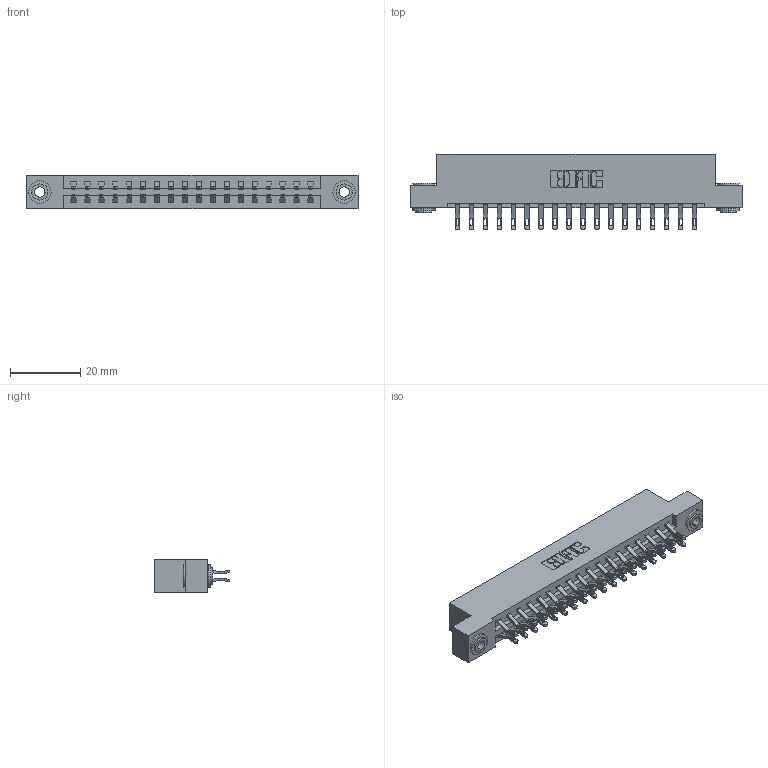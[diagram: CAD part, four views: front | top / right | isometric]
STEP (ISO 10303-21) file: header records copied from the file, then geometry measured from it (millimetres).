
FILE_DESCRIPTION (( 'STEP AP203' ), '1' );
FILE_NAME ('337-036-555-203.STEP', '2019-10-08T21:03:38', ( '' ), ( '' ), 'SwSTEP 2.0', 'SolidWorks 2016', '' );
FILE_SCHEMA (( 'CONFIG_CONTROL_DESIGN' ));
Length unit declared in the file: inch
Products named in the file (4): 345-292-001_555 Tail; 337 Part_Flush Mounting Lugs - 0.156 Dia-TH; 345-250-002_345-250-002-102; 337-036-555-203
Assembly tree (39 placements, depth 2):
  337-036-555-203
    337 Part_Flush Mounting Lugs - 0.156 Dia-TH
    345-292-001_555 Tail  x36
    345-250-002_345-250-002-102  x2
Bounding box: 94.34 x 21.47 x 9.4 mm (x, y, z)
Volume: 9746.2 mm3; surface area: 11402.9 mm2
Topology: 39 solids, 39 shells, 2312 faces, 7191 edges, 4790 vertices
Faces by surface type: plane 1376, cylinder 928, cone 8
Entity records: 18036 total; most frequent: CARTESIAN_POINT 3067, ORIENTED_EDGE 2966, DIRECTION 2657, EDGE_CURVE 1483, LINE 1311, VECTOR 1311, VERTEX_POINT 986, AXIS2_PLACEMENT_3D 673
